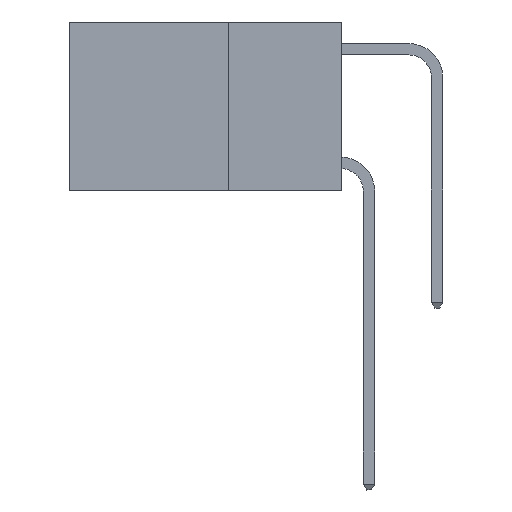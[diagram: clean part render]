
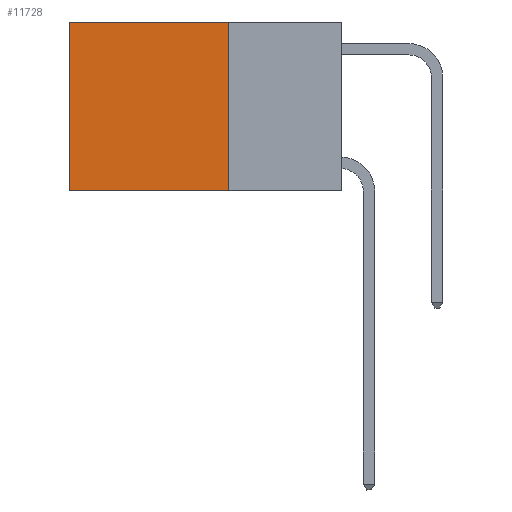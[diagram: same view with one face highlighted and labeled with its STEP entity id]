
A CAD part, left-side view. The second image highlights one B-rep face of the part: STEP entity #11728.
In plain terms, the highlighted planar face has unit normal (-1, 0, 0).
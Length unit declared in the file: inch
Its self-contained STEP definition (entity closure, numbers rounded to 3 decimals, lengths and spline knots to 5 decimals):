
#352 = DIRECTION ( 'NONE',  ( 0., 1., 0. ) ) ;
#1267 = FACE_OUTER_BOUND ( 'NONE', #11181, .T. ) ;
#1282 = VERTEX_POINT ( 'NONE', #11262 ) ;
#1302 = AXIS2_PLACEMENT_3D ( 'NONE', #5953, #10002, #3926 ) ;
#1465 = DIRECTION ( 'NONE',  ( 0., 0., -1. ) ) ;
#1923 = LINE ( 'NONE', #6603, #5032 ) ;
#2092 = LINE ( 'NONE', #9670, #7243 ) ;
#2435 = CARTESIAN_POINT ( 'NONE',  ( 0.2625, 0.25, 0. ) ) ;
#2881 = PLANE ( 'NONE',  #1302 ) ;
#3181 = VERTEX_POINT ( 'NONE', #5331 ) ;
#3926 = DIRECTION ( 'NONE',  ( 0., 0., -1. ) ) ;
#4585 = CARTESIAN_POINT ( 'NONE',  ( 0.2625, 0.25, -0.37 ) ) ;
#5032 = VECTOR ( 'NONE', #352, 39.37008 ) ;
#5331 = CARTESIAN_POINT ( 'NONE',  ( 0.2625, 0.6, 0. ) ) ;
#5953 = CARTESIAN_POINT ( 'NONE',  ( 0.2625, 0.25, 0. ) ) ;
#6342 = EDGE_CURVE ( 'NONE', #1282, #12899, #12686, .T. ) ;
#6603 = CARTESIAN_POINT ( 'NONE',  ( 0.2625, 0.25, -0.37 ) ) ;
#6707 = DIRECTION ( 'NONE',  ( 0., 1., 0. ) ) ;
#7007 = CARTESIAN_POINT ( 'NONE',  ( 0.2625, 0.6, -0.37 ) ) ;
#7243 = VECTOR ( 'NONE', #1465, 39.37008 ) ;
#7422 = VECTOR ( 'NONE', #10545, 39.37008 ) ;
#8838 = EDGE_CURVE ( 'NONE', #1282, #3181, #9893, .T. ) ;
#9058 = VERTEX_POINT ( 'NONE', #7007 ) ;
#9180 = ORIENTED_EDGE ( 'NONE', *, *, #12326, .T. ) ;
#9276 = ORIENTED_EDGE ( 'NONE', *, *, #12105, .F. ) ;
#9371 = ORIENTED_EDGE ( 'NONE', *, *, #6342, .F. ) ;
#9398 = ORIENTED_EDGE ( 'NONE', *, *, #8838, .T. ) ;
#9670 = CARTESIAN_POINT ( 'NONE',  ( 0.2625, 0.6, 0. ) ) ;
#9893 = LINE ( 'NONE', #12634, #12766 ) ;
#10002 = DIRECTION ( 'NONE',  ( 1., 0., 0. ) ) ;
#10545 = DIRECTION ( 'NONE',  ( 0., 0., -1. ) ) ;
#11181 = EDGE_LOOP ( 'NONE', ( #9180, #9276, #9371, #9398 ) ) ;
#11262 = CARTESIAN_POINT ( 'NONE',  ( 0.2625, 0.25, 0. ) ) ;
#11728 = ADVANCED_FACE ( 'NONE', ( #1267 ), #2881, .F. ) ;
#12105 = EDGE_CURVE ( 'NONE', #12899, #9058, #1923, .T. ) ;
#12326 = EDGE_CURVE ( 'NONE', #3181, #9058, #2092, .T. ) ;
#12634 = CARTESIAN_POINT ( 'NONE',  ( 0.2625, 0.25, 0. ) ) ;
#12686 = LINE ( 'NONE', #2435, #7422 ) ;
#12766 = VECTOR ( 'NONE', #6707, 39.37008 ) ;
#12899 = VERTEX_POINT ( 'NONE', #4585 ) ;
